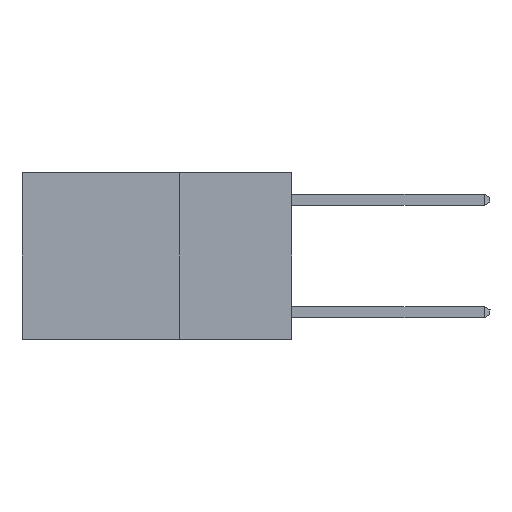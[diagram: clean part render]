
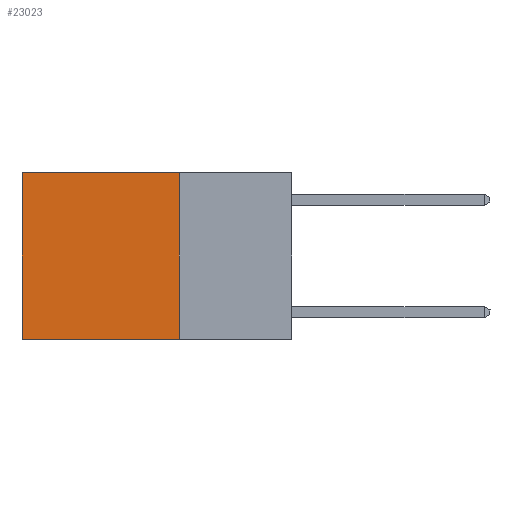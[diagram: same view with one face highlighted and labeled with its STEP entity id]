
A CAD part, left-side view. The second image highlights one B-rep face of the part: STEP entity #23023.
In plain terms, the highlighted planar face has unit normal (-1, 0, 0).
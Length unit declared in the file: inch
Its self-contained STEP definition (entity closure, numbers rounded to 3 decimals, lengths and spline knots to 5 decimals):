
#790 = CARTESIAN_POINT ( 'NONE',  ( 0.2625, 0.25, 0. ) ) ;
#872 = VECTOR ( 'NONE', #18218, 39.37008 ) ;
#2790 = ORIENTED_EDGE ( 'NONE', *, *, #8632, .F. ) ;
#2934 = CARTESIAN_POINT ( 'NONE',  ( 0.2625, 0.25, 0. ) ) ;
#4641 = EDGE_CURVE ( 'NONE', #24914, #9215, #24511, .T. ) ;
#4789 = DIRECTION ( 'NONE',  ( 0., 0., -1. ) ) ;
#5241 = LINE ( 'NONE', #18550, #22838 ) ;
#7363 = EDGE_CURVE ( 'NONE', #24914, #20240, #26474, .T. ) ;
#7999 = EDGE_CURVE ( 'NONE', #9215, #24215, #5241, .T. ) ;
#8632 = EDGE_CURVE ( 'NONE', #20240, #24215, #12438, .T. ) ;
#9215 = VERTEX_POINT ( 'NONE', #18000 ) ;
#9776 = FACE_OUTER_BOUND ( 'NONE', #13632, .T. ) ;
#10464 = ORIENTED_EDGE ( 'NONE', *, *, #7363, .F. ) ;
#10978 = ORIENTED_EDGE ( 'NONE', *, *, #4641, .T. ) ;
#12325 = VECTOR ( 'NONE', #23669, 39.37008 ) ;
#12396 = DIRECTION ( 'NONE',  ( 0., 0., -1. ) ) ;
#12438 = LINE ( 'NONE', #29495, #872 ) ;
#13632 = EDGE_LOOP ( 'NONE', ( #23134, #2790, #10464, #10978 ) ) ;
#14262 = VECTOR ( 'NONE', #15868, 39.37008 ) ;
#15868 = DIRECTION ( 'NONE',  ( 0., 0., -1. ) ) ;
#16650 = CARTESIAN_POINT ( 'NONE',  ( 0.2625, 0.6, -0.37 ) ) ;
#16721 = CARTESIAN_POINT ( 'NONE',  ( 0.2625, 0.25, 0. ) ) ;
#18000 = CARTESIAN_POINT ( 'NONE',  ( 0.2625, 0.6, 0. ) ) ;
#18218 = DIRECTION ( 'NONE',  ( 0., 1., 0. ) ) ;
#18550 = CARTESIAN_POINT ( 'NONE',  ( 0.2625, 0.6, 0. ) ) ;
#20240 = VERTEX_POINT ( 'NONE', #22441 ) ;
#20407 = CARTESIAN_POINT ( 'NONE',  ( 0.2625, 0.25, 0. ) ) ;
#22441 = CARTESIAN_POINT ( 'NONE',  ( 0.2625, 0.25, -0.37 ) ) ;
#22838 = VECTOR ( 'NONE', #4789, 39.37008 ) ;
#23023 = ADVANCED_FACE ( 'NONE', ( #9776 ), #23838, .F. ) ;
#23134 = ORIENTED_EDGE ( 'NONE', *, *, #7999, .T. ) ;
#23669 = DIRECTION ( 'NONE',  ( 0., 1., 0. ) ) ;
#23838 = PLANE ( 'NONE',  #23960 ) ;
#23960 = AXIS2_PLACEMENT_3D ( 'NONE', #790, #26078, #12396 ) ;
#24215 = VERTEX_POINT ( 'NONE', #16650 ) ;
#24511 = LINE ( 'NONE', #16721, #12325 ) ;
#24914 = VERTEX_POINT ( 'NONE', #2934 ) ;
#26078 = DIRECTION ( 'NONE',  ( 1., 0., 0. ) ) ;
#26474 = LINE ( 'NONE', #20407, #14262 ) ;
#29495 = CARTESIAN_POINT ( 'NONE',  ( 0.2625, 0.25, -0.37 ) ) ;
